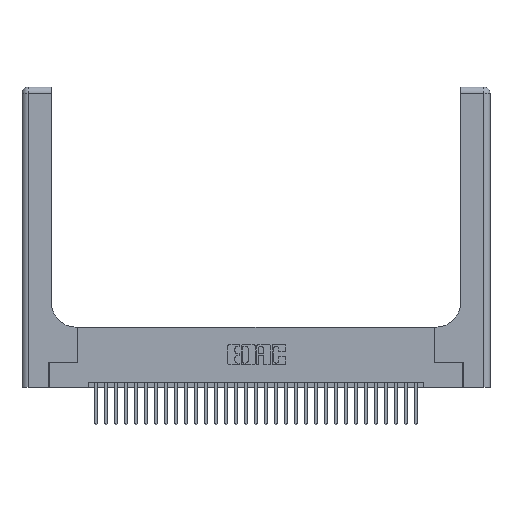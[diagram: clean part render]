
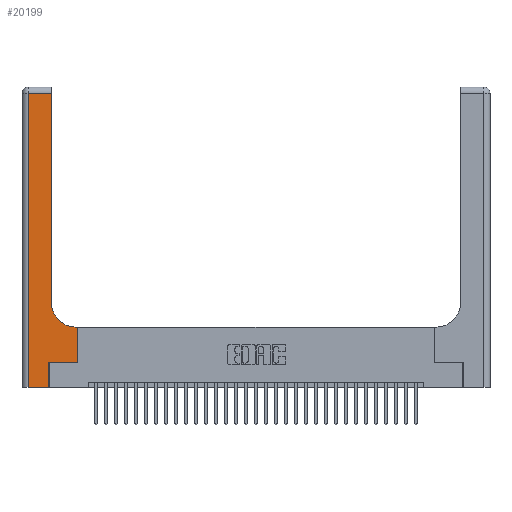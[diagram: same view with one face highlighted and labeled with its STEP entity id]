
A CAD part, top view. The second image highlights one B-rep face of the part: STEP entity #20199.
In plain terms, the highlighted planar face has unit normal (0, 0, 1).
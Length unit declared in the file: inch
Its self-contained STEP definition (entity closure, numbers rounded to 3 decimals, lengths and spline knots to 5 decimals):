
#467 = EDGE_CURVE ( 'NONE', #30186, #31078, #1347, .T. ) ;
#788 = LINE ( 'NONE', #9460, #1594 ) ;
#806 = VERTEX_POINT ( 'NONE', #20654 ) ;
#1347 = LINE ( 'NONE', #18970, #27128 ) ;
#1594 = VECTOR ( 'NONE', #29537, 39.37008 ) ;
#1711 = ORIENTED_EDGE ( 'NONE', *, *, #13337, .T. ) ;
#2051 = VERTEX_POINT ( 'NONE', #21406 ) ;
#2500 = DIRECTION ( 'NONE',  ( -1., 0., 0. ) ) ;
#2508 = AXIS2_PLACEMENT_3D ( 'NONE', #22210, #12222, #2500 ) ;
#2638 = ORIENTED_EDGE ( 'NONE', *, *, #27821, .T. ) ;
#2671 = VECTOR ( 'NONE', #27042, 39.37008 ) ;
#4225 = CARTESIAN_POINT ( 'NONE',  ( 0.5415, 0.85, 0.37 ) ) ;
#4494 = VERTEX_POINT ( 'NONE', #17327 ) ;
#5295 = VECTOR ( 'NONE', #22516, 39.37008 ) ;
#6982 = ORIENTED_EDGE ( 'NONE', *, *, #20630, .T. ) ;
#7334 = ORIENTED_EDGE ( 'NONE', *, *, #30600, .T. ) ;
#7756 = CARTESIAN_POINT ( 'NONE',  ( 0.06, 0., 0.37 ) ) ;
#8464 = LINE ( 'NONE', #8710, #29548 ) ;
#8710 = CARTESIAN_POINT ( 'NONE',  ( 0.5585, 0.25, 0.37 ) ) ;
#9460 = CARTESIAN_POINT ( 'NONE',  ( 0.06, 3., 0.37 ) ) ;
#9596 = CARTESIAN_POINT ( 'NONE',  ( 0.269, 0., 0.37 ) ) ;
#9961 = VERTEX_POINT ( 'NONE', #26847 ) ;
#11249 = ORIENTED_EDGE ( 'NONE', *, *, #25411, .T. ) ;
#11319 = DIRECTION ( 'NONE',  ( 0., 1., 0. ) ) ;
#11629 = DIRECTION ( 'NONE',  ( 0., 0., -1. ) ) ;
#11847 = ORIENTED_EDGE ( 'NONE', *, *, #467, .T. ) ;
#12222 = DIRECTION ( 'NONE',  ( 0., 0., -1. ) ) ;
#13337 = EDGE_CURVE ( 'NONE', #31078, #4494, #8464, .T. ) ;
#13520 = ORIENTED_EDGE ( 'NONE', *, *, #27125, .T. ) ;
#14028 = VERTEX_POINT ( 'NONE', #7756 ) ;
#14673 = CIRCLE ( 'NONE', #28279, 0.25 ) ;
#15237 = CARTESIAN_POINT ( 'NONE',  ( 0., 2.94, 0.37 ) ) ;
#16470 = FACE_OUTER_BOUND ( 'NONE', #19518, .T. ) ;
#16625 = DIRECTION ( 'NONE',  ( 1., 0., 0. ) ) ;
#16757 = EDGE_CURVE ( 'NONE', #806, #2051, #21467, .T. ) ;
#17071 = CARTESIAN_POINT ( 'NONE',  ( 0.2915, 0.6, 0.37 ) ) ;
#17321 = PLANE ( 'NONE',  #2508 ) ;
#17327 = CARTESIAN_POINT ( 'NONE',  ( 0.5585, 0.6, 0.37 ) ) ;
#18194 = LINE ( 'NONE', #22558, #28731 ) ;
#18202 = CARTESIAN_POINT ( 'NONE',  ( 0., 0., 0.37 ) ) ;
#18970 = CARTESIAN_POINT ( 'NONE',  ( 0.269, 0.25, 0.37 ) ) ;
#19133 = VERTEX_POINT ( 'NONE', #25744 ) ;
#19518 = EDGE_LOOP ( 'NONE', ( #27509, #2638, #7334, #6982, #13520, #11847, #1711, #25434, #11249 ) ) ;
#20199 = ADVANCED_FACE ( 'NONE', ( #16470 ), #17321, .F. ) ;
#20630 = EDGE_CURVE ( 'NONE', #14028, #29403, #30151, .T. ) ;
#20654 = CARTESIAN_POINT ( 'NONE',  ( 0.2915, 0.85, 0.37 ) ) ;
#20708 = DIRECTION ( 'NONE',  ( 0., 1., 0. ) ) ;
#20719 = DIRECTION ( 'NONE',  ( 1., 0., 0. ) ) ;
#21406 = CARTESIAN_POINT ( 'NONE',  ( 0.2915, 2.94, 0.37 ) ) ;
#21467 = LINE ( 'NONE', #30970, #31648 ) ;
#22210 = CARTESIAN_POINT ( 'NONE',  ( 0., 3., 0.37 ) ) ;
#22516 = DIRECTION ( 'NONE',  ( -1., 0., 0. ) ) ;
#22558 = CARTESIAN_POINT ( 'NONE',  ( 0.269, 0., 0.37 ) ) ;
#23529 = EDGE_CURVE ( 'NONE', #4494, #9961, #28824, .T. ) ;
#25191 = DIRECTION ( 'NONE',  ( 0., 1., 0. ) ) ;
#25411 = EDGE_CURVE ( 'NONE', #9961, #806, #14673, .T. ) ;
#25434 = ORIENTED_EDGE ( 'NONE', *, *, #23529, .T. ) ;
#25744 = CARTESIAN_POINT ( 'NONE',  ( 0.06, 2.94, 0.37 ) ) ;
#26847 = CARTESIAN_POINT ( 'NONE',  ( 0.5415, 0.6, 0.37 ) ) ;
#26885 = CARTESIAN_POINT ( 'NONE',  ( 0.5585, 0.25, 0.37 ) ) ;
#27042 = DIRECTION ( 'NONE',  ( -1., 0., 0. ) ) ;
#27125 = EDGE_CURVE ( 'NONE', #29403, #30186, #18194, .T. ) ;
#27128 = VECTOR ( 'NONE', #29111, 39.37008 ) ;
#27509 = ORIENTED_EDGE ( 'NONE', *, *, #16757, .T. ) ;
#27821 = EDGE_CURVE ( 'NONE', #2051, #19133, #28701, .T. ) ;
#28279 = AXIS2_PLACEMENT_3D ( 'NONE', #4225, #11629, #16625 ) ;
#28701 = LINE ( 'NONE', #15237, #5295 ) ;
#28731 = VECTOR ( 'NONE', #25191, 39.37008 ) ;
#28824 = LINE ( 'NONE', #17071, #2671 ) ;
#29111 = DIRECTION ( 'NONE',  ( 1., 0., 0. ) ) ;
#29403 = VERTEX_POINT ( 'NONE', #9596 ) ;
#29537 = DIRECTION ( 'NONE',  ( 0., -1., 0. ) ) ;
#29548 = VECTOR ( 'NONE', #11319, 39.37008 ) ;
#30151 = LINE ( 'NONE', #18202, #30913 ) ;
#30186 = VERTEX_POINT ( 'NONE', #30626 ) ;
#30600 = EDGE_CURVE ( 'NONE', #19133, #14028, #788, .T. ) ;
#30626 = CARTESIAN_POINT ( 'NONE',  ( 0.269, 0.25, 0.37 ) ) ;
#30913 = VECTOR ( 'NONE', #20719, 39.37008 ) ;
#30970 = CARTESIAN_POINT ( 'NONE',  ( 0.2915, 3., 0.37 ) ) ;
#31078 = VERTEX_POINT ( 'NONE', #26885 ) ;
#31648 = VECTOR ( 'NONE', #20708, 39.37008 ) ;
